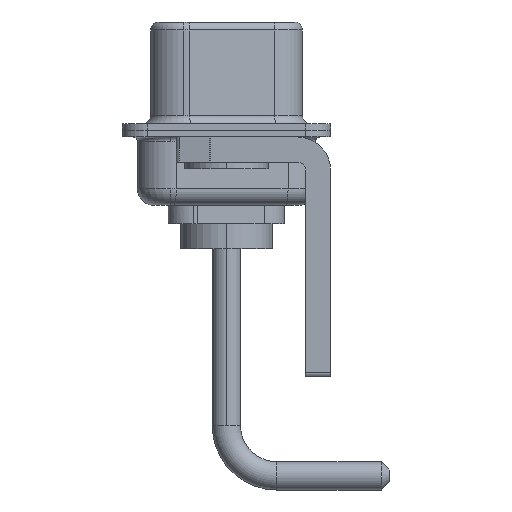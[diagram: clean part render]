
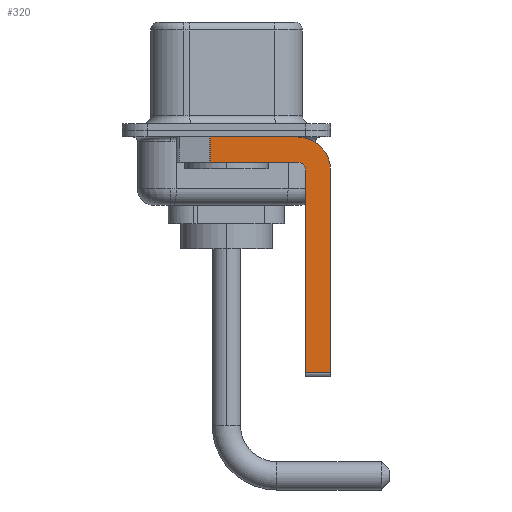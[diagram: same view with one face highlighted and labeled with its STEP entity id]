
A CAD part, left-side view. The second image highlights one B-rep face of the part: STEP entity #320.
In plain terms, the highlighted planar face has unit normal (-1, 0, 0).
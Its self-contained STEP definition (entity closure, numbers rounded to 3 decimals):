
#99 = VECTOR ( 'NONE', #5063, 1000. ) ;
#291 = CARTESIAN_POINT ( 'NONE',  ( -2.9, 0.978, -1.9 ) ) ;
#320 = ADVANCED_FACE ( 'NONE', ( #13971 ), #15123, .F. ) ;
#379 = EDGE_CURVE ( 'NONE', #14468, #8139, #8300, .T. ) ;
#859 = LINE ( 'NONE', #11353, #7168 ) ;
#1009 = CARTESIAN_POINT ( 'NONE',  ( -2.9, 3., -0.4 ) ) ;
#1013 = EDGE_LOOP ( 'NONE', ( #10476, #13233, #1230, #14480, #2711, #2738, #4911, #7898 ) ) ;
#1216 = VECTOR ( 'NONE', #12733, 1000. ) ;
#1230 = ORIENTED_EDGE ( 'NONE', *, *, #14389, .F. ) ;
#1311 = CIRCLE ( 'NONE', #9631, 2. ) ;
#1889 = AXIS2_PLACEMENT_3D ( 'NONE', #12585, #2091, #10361 ) ;
#2053 = CARTESIAN_POINT ( 'NONE',  ( -2.9, -4.25, -1.9 ) ) ;
#2091 = DIRECTION ( 'NONE',  ( -1., 0., 0. ) ) ;
#2317 = CARTESIAN_POINT ( 'NONE',  ( -2.9, -4.25, -0.4 ) ) ;
#2711 = ORIENTED_EDGE ( 'NONE', *, *, #379, .F. ) ;
#2738 = ORIENTED_EDGE ( 'NONE', *, *, #5397, .T. ) ;
#2890 = CARTESIAN_POINT ( 'NONE',  ( -2.9, -6.25, -14.55 ) ) ;
#2967 = CARTESIAN_POINT ( 'NONE',  ( -2.9, -4.25, -2.4 ) ) ;
#3279 = CARTESIAN_POINT ( 'NONE',  ( -2.9, -4.75, -14.55 ) ) ;
#3328 = LINE ( 'NONE', #5629, #5136 ) ;
#3707 = LINE ( 'NONE', #3943, #11601 ) ;
#3943 = CARTESIAN_POINT ( 'NONE',  ( -2.9, 0.978, -1.9 ) ) ;
#4181 = EDGE_CURVE ( 'NONE', #10191, #6671, #859, .T. ) ;
#4288 = CARTESIAN_POINT ( 'NONE',  ( -2.9, 0.978, -0.4 ) ) ;
#4440 = DIRECTION ( 'NONE',  ( 0., 0., -1. ) ) ;
#4522 = DIRECTION ( 'NONE',  ( 0., 0., -1. ) ) ;
#4603 = DIRECTION ( 'NONE',  ( 1., 0., 0. ) ) ;
#4608 = CARTESIAN_POINT ( 'NONE',  ( -2.9, -4.75, -2.4 ) ) ;
#4746 = CARTESIAN_POINT ( 'NONE',  ( -2.9, -6.25, -2.4 ) ) ;
#4911 = ORIENTED_EDGE ( 'NONE', *, *, #4181, .F. ) ;
#5063 = DIRECTION ( 'NONE',  ( 0., -1., 0. ) ) ;
#5136 = VECTOR ( 'NONE', #7861, 1000. ) ;
#5397 = EDGE_CURVE ( 'NONE', #14468, #6671, #3328, .T. ) ;
#5629 = CARTESIAN_POINT ( 'NONE',  ( -2.9, -4.25, -14.55 ) ) ;
#6671 = VERTEX_POINT ( 'NONE', #2890 ) ;
#6916 = CARTESIAN_POINT ( 'NONE',  ( -2.9, -4.25, -2.4 ) ) ;
#7168 = VECTOR ( 'NONE', #4522, 1000. ) ;
#7337 = DIRECTION ( 'NONE',  ( 0., 0., -1. ) ) ;
#7465 = EDGE_CURVE ( 'NONE', #8139, #10236, #7531, .T. ) ;
#7531 = CIRCLE ( 'NONE', #1889, 0.5 ) ;
#7770 = VECTOR ( 'NONE', #11621, 1000. ) ;
#7861 = DIRECTION ( 'NONE',  ( 0., -1., 0. ) ) ;
#7898 = ORIENTED_EDGE ( 'NONE', *, *, #10703, .F. ) ;
#8049 = VERTEX_POINT ( 'NONE', #291 ) ;
#8139 = VERTEX_POINT ( 'NONE', #4608 ) ;
#8300 = LINE ( 'NONE', #14048, #1216 ) ;
#8659 = VERTEX_POINT ( 'NONE', #4288 ) ;
#9631 = AXIS2_PLACEMENT_3D ( 'NONE', #2967, #9942, #12085 ) ;
#9942 = DIRECTION ( 'NONE',  ( 1., 0., 0. ) ) ;
#10191 = VERTEX_POINT ( 'NONE', #4746 ) ;
#10236 = VERTEX_POINT ( 'NONE', #11118 ) ;
#10361 = DIRECTION ( 'NONE',  ( 0., 0., 1. ) ) ;
#10476 = ORIENTED_EDGE ( 'NONE', *, *, #11540, .F. ) ;
#10529 = LINE ( 'NONE', #1009, #99 ) ;
#10703 = EDGE_CURVE ( 'NONE', #12967, #10191, #1311, .T. ) ;
#11118 = CARTESIAN_POINT ( 'NONE',  ( -2.9, -4.25, -1.9 ) ) ;
#11353 = CARTESIAN_POINT ( 'NONE',  ( -2.9, -6.25, -2.4 ) ) ;
#11491 = AXIS2_PLACEMENT_3D ( 'NONE', #6916, #4603, #4440 ) ;
#11540 = EDGE_CURVE ( 'NONE', #8659, #12967, #10529, .T. ) ;
#11601 = VECTOR ( 'NONE', #7337, 1000. ) ;
#11621 = DIRECTION ( 'NONE',  ( 0., 1., 0. ) ) ;
#12085 = DIRECTION ( 'NONE',  ( 0., 0., -1. ) ) ;
#12153 = EDGE_CURVE ( 'NONE', #8659, #8049, #3707, .T. ) ;
#12543 = LINE ( 'NONE', #2053, #7770 ) ;
#12585 = CARTESIAN_POINT ( 'NONE',  ( -2.9, -4.25, -2.4 ) ) ;
#12733 = DIRECTION ( 'NONE',  ( 0., 0., 1. ) ) ;
#12967 = VERTEX_POINT ( 'NONE', #2317 ) ;
#13233 = ORIENTED_EDGE ( 'NONE', *, *, #12153, .T. ) ;
#13971 = FACE_OUTER_BOUND ( 'NONE', #1013, .T. ) ;
#14048 = CARTESIAN_POINT ( 'NONE',  ( -2.9, -4.75, -14.8 ) ) ;
#14389 = EDGE_CURVE ( 'NONE', #10236, #8049, #12543, .T. ) ;
#14468 = VERTEX_POINT ( 'NONE', #3279 ) ;
#14480 = ORIENTED_EDGE ( 'NONE', *, *, #7465, .F. ) ;
#15123 = PLANE ( 'NONE',  #11491 ) ;
